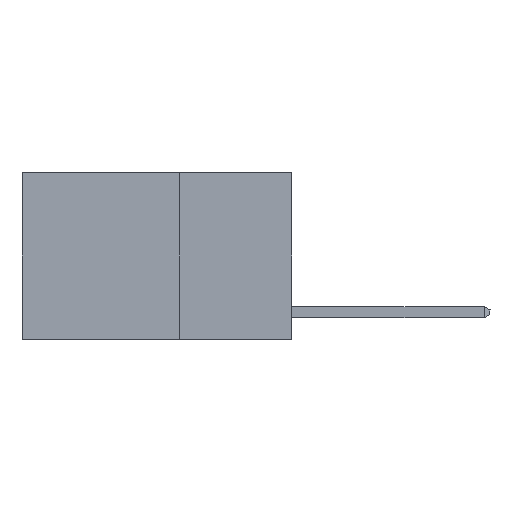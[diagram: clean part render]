
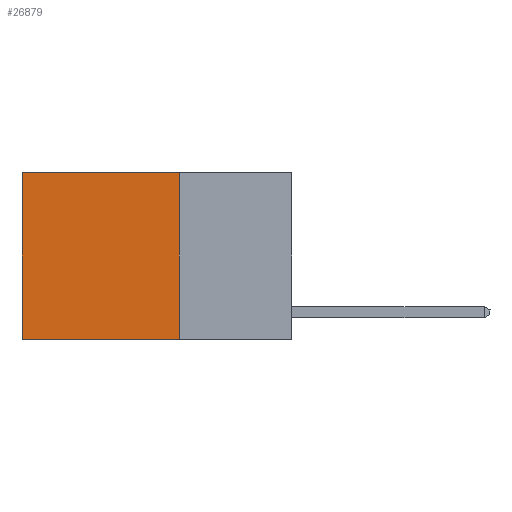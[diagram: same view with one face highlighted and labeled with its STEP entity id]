
A CAD part, left-side view. The second image highlights one B-rep face of the part: STEP entity #26879.
In plain terms, the highlighted planar face has unit normal (-1, 0, 0).
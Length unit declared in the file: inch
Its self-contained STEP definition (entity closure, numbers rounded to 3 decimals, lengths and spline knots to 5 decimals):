
#74 = LINE ( 'NONE', #18286, #23947 ) ;
#601 = DIRECTION ( 'NONE',  ( 0., 1., 0. ) ) ;
#977 = ORIENTED_EDGE ( 'NONE', *, *, #25486, .F. ) ;
#1635 = DIRECTION ( 'NONE',  ( 0., 0., -1. ) ) ;
#2070 = VECTOR ( 'NONE', #1635, 39.37008 ) ;
#2647 = CARTESIAN_POINT ( 'NONE',  ( 0.2625, 0.25, 0. ) ) ;
#3528 = VECTOR ( 'NONE', #23039, 39.37008 ) ;
#4782 = DIRECTION ( 'NONE',  ( 1., 0., 0. ) ) ;
#7278 = LINE ( 'NONE', #16633, #3528 ) ;
#7298 = EDGE_CURVE ( 'NONE', #23224, #24645, #74, .T. ) ;
#7394 = CARTESIAN_POINT ( 'NONE',  ( 0.2625, 0.25, 0. ) ) ;
#9069 = CARTESIAN_POINT ( 'NONE',  ( 0.2625, 0.25, -0.37 ) ) ;
#9104 = PLANE ( 'NONE',  #24007 ) ;
#9117 = ORIENTED_EDGE ( 'NONE', *, *, #19837, .T. ) ;
#9247 = CARTESIAN_POINT ( 'NONE',  ( 0.2625, 0.6, -0.37 ) ) ;
#10265 = VERTEX_POINT ( 'NONE', #9247 ) ;
#11045 = ORIENTED_EDGE ( 'NONE', *, *, #7298, .F. ) ;
#11053 = VERTEX_POINT ( 'NONE', #11562 ) ;
#11562 = CARTESIAN_POINT ( 'NONE',  ( 0.2625, 0.6, 0. ) ) ;
#13924 = DIRECTION ( 'NONE',  ( 0., 0., -1. ) ) ;
#14548 = ORIENTED_EDGE ( 'NONE', *, *, #18939, .T. ) ;
#15884 = DIRECTION ( 'NONE',  ( 0., 0., -1. ) ) ;
#16633 = CARTESIAN_POINT ( 'NONE',  ( 0.2625, 0.25, -0.37 ) ) ;
#17216 = EDGE_LOOP ( 'NONE', ( #14548, #977, #11045, #9117 ) ) ;
#18286 = CARTESIAN_POINT ( 'NONE',  ( 0.2625, 0.25, 0. ) ) ;
#18939 = EDGE_CURVE ( 'NONE', #11053, #10265, #27333, .T. ) ;
#19432 = VECTOR ( 'NONE', #601, 39.37008 ) ;
#19837 = EDGE_CURVE ( 'NONE', #23224, #11053, #25234, .T. ) ;
#23039 = DIRECTION ( 'NONE',  ( 0., 1., 0. ) ) ;
#23224 = VERTEX_POINT ( 'NONE', #2647 ) ;
#23947 = VECTOR ( 'NONE', #13924, 39.37008 ) ;
#24007 = AXIS2_PLACEMENT_3D ( 'NONE', #24568, #4782, #15884 ) ;
#24568 = CARTESIAN_POINT ( 'NONE',  ( 0.2625, 0.25, 0. ) ) ;
#24645 = VERTEX_POINT ( 'NONE', #9069 ) ;
#24910 = FACE_OUTER_BOUND ( 'NONE', #17216, .T. ) ;
#25234 = LINE ( 'NONE', #7394, #19432 ) ;
#25486 = EDGE_CURVE ( 'NONE', #24645, #10265, #7278, .T. ) ;
#26068 = CARTESIAN_POINT ( 'NONE',  ( 0.2625, 0.6, 0. ) ) ;
#26879 = ADVANCED_FACE ( 'NONE', ( #24910 ), #9104, .F. ) ;
#27333 = LINE ( 'NONE', #26068, #2070 ) ;
